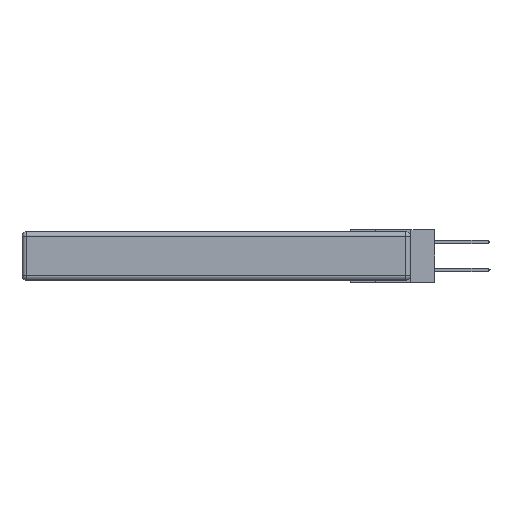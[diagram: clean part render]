
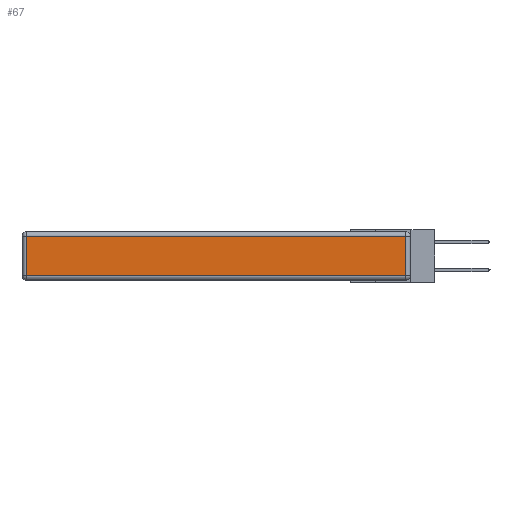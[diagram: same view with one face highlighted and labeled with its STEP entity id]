
A CAD part, left-side view. The second image highlights one B-rep face of the part: STEP entity #67.
In plain terms, the highlighted planar face has unit normal (-1, 0, 0).
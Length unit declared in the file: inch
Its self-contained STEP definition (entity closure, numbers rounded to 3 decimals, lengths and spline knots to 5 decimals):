
#16 = VERTEX_POINT ( 'NONE', #577 ) ;
#67 = ADVANCED_FACE ( 'NONE', ( #12036 ), #11786, .T. ) ;
#253 = LINE ( 'NONE', #1676, #4608 ) ;
#577 = CARTESIAN_POINT ( 'NONE',  ( 0., 2.72, -0.313 ) ) ;
#1019 = VERTEX_POINT ( 'NONE', #11197 ) ;
#1050 = VERTEX_POINT ( 'NONE', #4414 ) ;
#1676 = CARTESIAN_POINT ( 'NONE',  ( 0., 0.03, -0.343 ) ) ;
#1799 = DIRECTION ( 'NONE',  ( 0., 0., -1. ) ) ;
#2033 = DIRECTION ( 'NONE',  ( 0., 0., 1. ) ) ;
#2083 = LINE ( 'NONE', #9722, #3782 ) ;
#2312 = DIRECTION ( 'NONE',  ( 0., -1., 0. ) ) ;
#2440 = VECTOR ( 'NONE', #11081, 39.37008 ) ;
#3246 = ORIENTED_EDGE ( 'NONE', *, *, #12678, .T. ) ;
#3782 = VECTOR ( 'NONE', #1799, 39.37008 ) ;
#3839 = DIRECTION ( 'NONE',  ( -1., 0., 0. ) ) ;
#4392 = EDGE_CURVE ( 'NONE', #1019, #1050, #253, .T. ) ;
#4414 = CARTESIAN_POINT ( 'NONE',  ( 0., 0.03, -0.03 ) ) ;
#4608 = VECTOR ( 'NONE', #2033, 39.37008 ) ;
#5113 = VECTOR ( 'NONE', #2312, 39.37008 ) ;
#5201 = CARTESIAN_POINT ( 'NONE',  ( 0., 2.75, -0.03 ) ) ;
#5310 = EDGE_CURVE ( 'NONE', #1050, #9486, #12819, .T. ) ;
#5928 = ORIENTED_EDGE ( 'NONE', *, *, #5310, .T. ) ;
#6380 = CARTESIAN_POINT ( 'NONE',  ( 0., 0., -0.313 ) ) ;
#6486 = EDGE_CURVE ( 'NONE', #9486, #16, #2083, .T. ) ;
#6504 = LINE ( 'NONE', #6380, #5113 ) ;
#6769 = DIRECTION ( 'NONE',  ( 0., 0., 1. ) ) ;
#6935 = CARTESIAN_POINT ( 'NONE',  ( 0., 2.72, -0.03 ) ) ;
#8786 = CARTESIAN_POINT ( 'NONE',  ( 0., 0., -0.343 ) ) ;
#8973 = ORIENTED_EDGE ( 'NONE', *, *, #6486, .T. ) ;
#9347 = EDGE_LOOP ( 'NONE', ( #3246, #11766, #5928, #8973 ) ) ;
#9486 = VERTEX_POINT ( 'NONE', #6935 ) ;
#9722 = CARTESIAN_POINT ( 'NONE',  ( 0., 2.72, -0.343 ) ) ;
#10949 = AXIS2_PLACEMENT_3D ( 'NONE', #8786, #3839, #6769 ) ;
#11081 = DIRECTION ( 'NONE',  ( 0., 1., 0. ) ) ;
#11197 = CARTESIAN_POINT ( 'NONE',  ( 0., 0.03, -0.313 ) ) ;
#11766 = ORIENTED_EDGE ( 'NONE', *, *, #4392, .T. ) ;
#11786 = PLANE ( 'NONE',  #10949 ) ;
#12036 = FACE_OUTER_BOUND ( 'NONE', #9347, .T. ) ;
#12678 = EDGE_CURVE ( 'NONE', #16, #1019, #6504, .T. ) ;
#12819 = LINE ( 'NONE', #5201, #2440 ) ;
